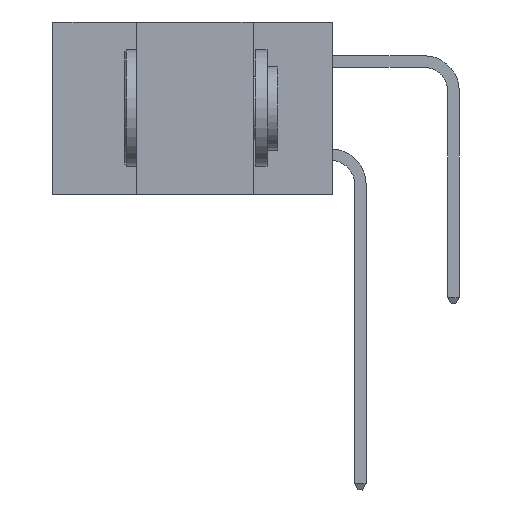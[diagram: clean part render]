
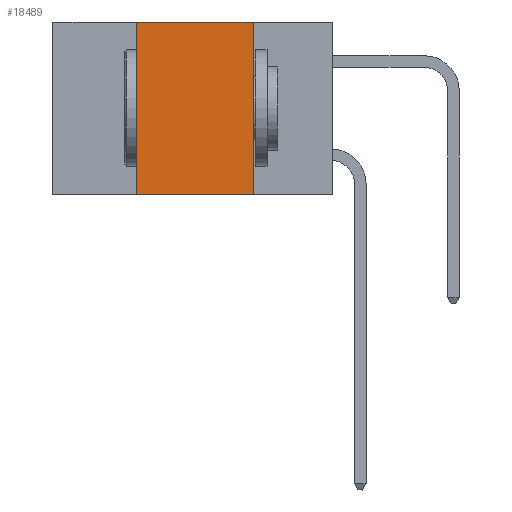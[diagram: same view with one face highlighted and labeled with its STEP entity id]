
A CAD part, left-side view. The second image highlights one B-rep face of the part: STEP entity #18489.
In plain terms, the highlighted planar face has unit normal (-1, 0, 0).
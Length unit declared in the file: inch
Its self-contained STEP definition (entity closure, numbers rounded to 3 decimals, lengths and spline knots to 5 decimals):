
#70 = CARTESIAN_POINT ( 'NONE',  ( 0., 0.6, -0.37 ) ) ;
#226 = CARTESIAN_POINT ( 'NONE',  ( 0., 0.42, 0. ) ) ;
#2506 = LINE ( 'NONE', #70, #5525 ) ;
#4376 = PLANE ( 'NONE',  #12191 ) ;
#4894 = CARTESIAN_POINT ( 'NONE',  ( 0., 0.42, -0.37 ) ) ;
#5161 = DIRECTION ( 'NONE',  ( 0., 0., -1. ) ) ;
#5525 = VECTOR ( 'NONE', #23186, 39.37008 ) ;
#5909 = CARTESIAN_POINT ( 'NONE',  ( 0., 0.6, 0. ) ) ;
#6321 = VERTEX_POINT ( 'NONE', #19927 ) ;
#6967 = LINE ( 'NONE', #10985, #23814 ) ;
#7154 = CARTESIAN_POINT ( 'NONE',  ( 0., 0.42, 0. ) ) ;
#8249 = ORIENTED_EDGE ( 'NONE', *, *, #23797, .F. ) ;
#9048 = VECTOR ( 'NONE', #17484, 39.37008 ) ;
#10622 = EDGE_CURVE ( 'NONE', #16303, #22167, #2506, .T. ) ;
#10884 = VERTEX_POINT ( 'NONE', #226 ) ;
#10985 = CARTESIAN_POINT ( 'NONE',  ( 0., 0.17, 0. ) ) ;
#11761 = LINE ( 'NONE', #7154, #22797 ) ;
#11896 = DIRECTION ( 'NONE',  ( 0., 0., -1. ) ) ;
#12191 = AXIS2_PLACEMENT_3D ( 'NONE', #17784, #15874, #11896 ) ;
#13482 = ORIENTED_EDGE ( 'NONE', *, *, #10622, .T. ) ;
#13509 = FACE_OUTER_BOUND ( 'NONE', #23323, .T. ) ;
#14052 = CARTESIAN_POINT ( 'NONE',  ( 0., 0.17, -0.37 ) ) ;
#14158 = LINE ( 'NONE', #5909, #9048 ) ;
#14858 = ORIENTED_EDGE ( 'NONE', *, *, #18117, .F. ) ;
#15874 = DIRECTION ( 'NONE',  ( 1., 0., 0. ) ) ;
#16303 = VERTEX_POINT ( 'NONE', #4894 ) ;
#17484 = DIRECTION ( 'NONE',  ( 0., -1., 0. ) ) ;
#17784 = CARTESIAN_POINT ( 'NONE',  ( 0., 0.6, 0. ) ) ;
#18117 = EDGE_CURVE ( 'NONE', #16303, #10884, #11761, .T. ) ;
#18489 = ADVANCED_FACE ( 'NONE', ( #13509 ), #4376, .F. ) ;
#19513 = EDGE_CURVE ( 'NONE', #6321, #22167, #6967, .T. ) ;
#19927 = CARTESIAN_POINT ( 'NONE',  ( 0., 0.17, 0. ) ) ;
#20259 = DIRECTION ( 'NONE',  ( 0., 0., 1. ) ) ;
#20833 = ORIENTED_EDGE ( 'NONE', *, *, #19513, .F. ) ;
#22167 = VERTEX_POINT ( 'NONE', #14052 ) ;
#22797 = VECTOR ( 'NONE', #20259, 39.37008 ) ;
#23186 = DIRECTION ( 'NONE',  ( 0., -1., 0. ) ) ;
#23323 = EDGE_LOOP ( 'NONE', ( #20833, #8249, #14858, #13482 ) ) ;
#23797 = EDGE_CURVE ( 'NONE', #10884, #6321, #14158, .T. ) ;
#23814 = VECTOR ( 'NONE', #5161, 39.37008 ) ;
